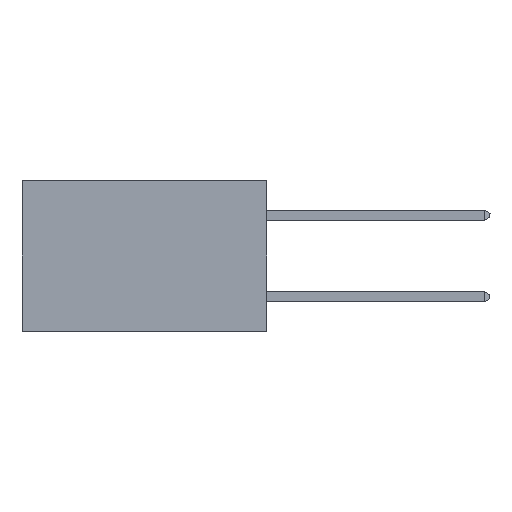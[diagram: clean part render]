
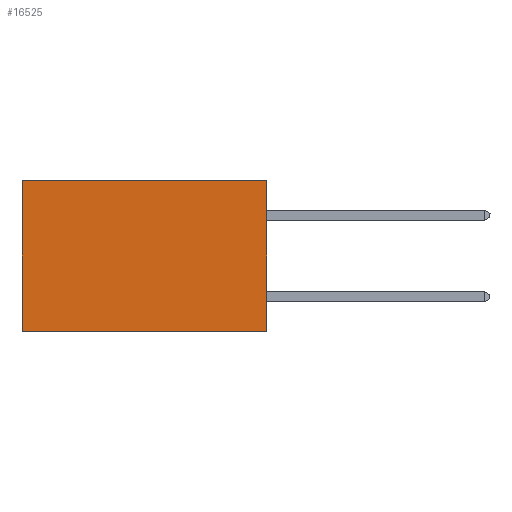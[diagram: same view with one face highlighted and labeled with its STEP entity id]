
A CAD part, left-side view. The second image highlights one B-rep face of the part: STEP entity #16525.
In plain terms, the highlighted planar face has unit normal (-1, 0, 0).
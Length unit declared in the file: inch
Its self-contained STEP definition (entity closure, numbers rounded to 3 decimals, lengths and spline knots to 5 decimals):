
#20 = ORIENTED_EDGE ( 'NONE', *, *, #25565, .F. ) ;
#2854 = CARTESIAN_POINT ( 'NONE',  ( 0.2875, 0., 0. ) ) ;
#3429 = EDGE_CURVE ( 'NONE', #12187, #14939, #29118, .T. ) ;
#4350 = DIRECTION ( 'NONE',  ( 0., 0., -1. ) ) ;
#4826 = LINE ( 'NONE', #27301, #29985 ) ;
#5249 = EDGE_CURVE ( 'NONE', #22240, #12187, #4826, .T. ) ;
#5729 = AXIS2_PLACEMENT_3D ( 'NONE', #18299, #22190, #25543 ) ;
#7879 = CARTESIAN_POINT ( 'NONE',  ( 0.2875, 0., -0.37 ) ) ;
#10688 = CARTESIAN_POINT ( 'NONE',  ( 0.2875, 0.6, -0.37 ) ) ;
#10741 = EDGE_LOOP ( 'NONE', ( #29541, #14192, #20, #19347 ) ) ;
#10879 = DIRECTION ( 'NONE',  ( 0., 0., -1. ) ) ;
#11309 = CARTESIAN_POINT ( 'NONE',  ( 0.2875, 0., -0.37 ) ) ;
#11857 = PLANE ( 'NONE',  #5729 ) ;
#12187 = VERTEX_POINT ( 'NONE', #40900 ) ;
#14192 = ORIENTED_EDGE ( 'NONE', *, *, #39277, .F. ) ;
#14768 = DIRECTION ( 'NONE',  ( 0., 1., 0. ) ) ;
#14939 = VERTEX_POINT ( 'NONE', #10688 ) ;
#15924 = LINE ( 'NONE', #16881, #40590 ) ;
#15949 = LINE ( 'NONE', #11309, #25241 ) ;
#16525 = ADVANCED_FACE ( 'NONE', ( #38013 ), #11857, .F. ) ;
#16881 = CARTESIAN_POINT ( 'NONE',  ( 0.2875, 0., 0. ) ) ;
#18299 = CARTESIAN_POINT ( 'NONE',  ( 0.2875, 0., 0. ) ) ;
#19093 = VERTEX_POINT ( 'NONE', #7879 ) ;
#19269 = VECTOR ( 'NONE', #10879, 39.37008 ) ;
#19347 = ORIENTED_EDGE ( 'NONE', *, *, #5249, .T. ) ;
#22190 = DIRECTION ( 'NONE',  ( 1., 0., 0. ) ) ;
#22240 = VERTEX_POINT ( 'NONE', #2854 ) ;
#25241 = VECTOR ( 'NONE', #14768, 39.37008 ) ;
#25543 = DIRECTION ( 'NONE',  ( 0., 0., -1. ) ) ;
#25565 = EDGE_CURVE ( 'NONE', #22240, #19093, #15924, .T. ) ;
#27301 = CARTESIAN_POINT ( 'NONE',  ( 0.2875, 0., 0. ) ) ;
#29118 = LINE ( 'NONE', #33476, #19269 ) ;
#29541 = ORIENTED_EDGE ( 'NONE', *, *, #3429, .T. ) ;
#29985 = VECTOR ( 'NONE', #34324, 39.37008 ) ;
#33476 = CARTESIAN_POINT ( 'NONE',  ( 0.2875, 0.6, 0. ) ) ;
#34324 = DIRECTION ( 'NONE',  ( 0., 1., 0. ) ) ;
#38013 = FACE_OUTER_BOUND ( 'NONE', #10741, .T. ) ;
#39277 = EDGE_CURVE ( 'NONE', #19093, #14939, #15949, .T. ) ;
#40590 = VECTOR ( 'NONE', #4350, 39.37008 ) ;
#40900 = CARTESIAN_POINT ( 'NONE',  ( 0.2875, 0.6, 0. ) ) ;
